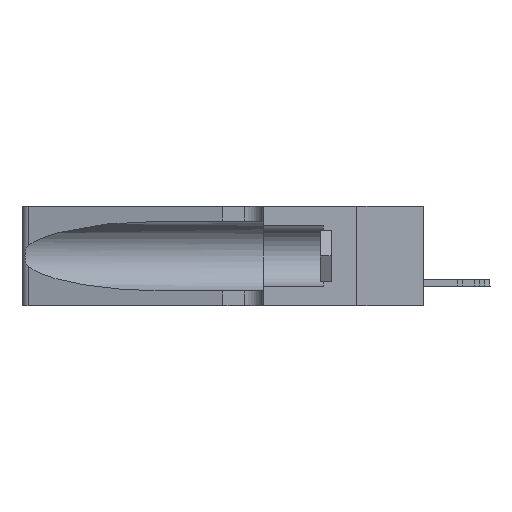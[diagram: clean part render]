
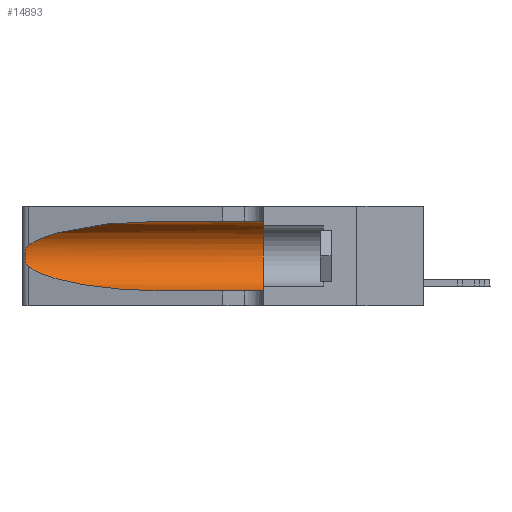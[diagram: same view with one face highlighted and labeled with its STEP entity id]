
A CAD part, left-side view. The second image highlights one B-rep face of the part: STEP entity #14893.
In plain terms, the highlighted cylindrical face has radius 3.308 mm (diameter 6.617 mm), a partial arc.
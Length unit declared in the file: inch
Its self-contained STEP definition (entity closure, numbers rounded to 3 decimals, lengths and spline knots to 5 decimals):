
#311 = ORIENTED_EDGE ( 'NONE', *, *, #1356, .T. ) ;
#380 = CARTESIAN_POINT ( 'NONE',  ( 0.1305, 1.61858, 0.185 ) ) ;
#923 = EDGE_CURVE ( 'NONE', #6857, #23272, #39423, .T. ) ;
#958 = VERTEX_POINT ( 'NONE', #23315 ) ;
#1293 = CARTESIAN_POINT ( 'NONE',  ( 0.25639, 1.23184, 0.21858 ) ) ;
#1356 = EDGE_CURVE ( 'NONE', #19249, #958, #8495, .T. ) ;
#1439 = CARTESIAN_POINT ( 'NONE',  ( 0.26018, 1.23835, 0.19895 ) ) ;
#3651 = CARTESIAN_POINT ( 'NONE',  ( 0.2373, 1.15595, 0.08982 ) ) ;
#4708 = CARTESIAN_POINT ( 'NONE',  ( 0.25787, 1.23484, 0.2124 ) ) ;
#4709 = ORIENTED_EDGE ( 'NONE', *, *, #27691, .F. ) ;
#4855 = CARTESIAN_POINT ( 'NONE',  ( 0.25856, 1.23593, 0.16098 ) ) ;
#5745 =( BOUNDED_CURVE ( )  B_SPLINE_CURVE ( 3, ( #30247, #43987, #16839, #43677 ),
 .UNSPECIFIED., .F., .F. ) 
 B_SPLINE_CURVE_WITH_KNOTS ( ( 4, 4 ),
 ( 1.5708, 2.84003 ),
 .UNSPECIFIED. ) 
 CURVE ( )  GEOMETRIC_REPRESENTATION_ITEM ( )  RATIONAL_B_SPLINE_CURVE ( ( 1., 0.87, 0.87, 1. ) ) 
 REPRESENTATION_ITEM ( '' )  );
#5772 = CYLINDRICAL_SURFACE ( 'NONE', #13787, 0.13025 ) ;
#6790 = CARTESIAN_POINT ( 'NONE',  ( 0.18966, 0.96281, 0.05475 ) ) ;
#6857 = VERTEX_POINT ( 'NONE', #15910 ) ;
#8495 =( BOUNDED_CURVE ( )  B_SPLINE_CURVE ( 3, ( #20632, #3651, #6790, #37813 ),
 .UNSPECIFIED., .F., .T. ) 
 B_SPLINE_CURVE_WITH_KNOTS ( ( 4, 4 ),
 ( 3.44316, 4.71239 ),
 .UNSPECIFIED. ) 
 CURVE ( )  GEOMETRIC_REPRESENTATION_ITEM ( )  RATIONAL_B_SPLINE_CURVE ( ( 1., 0.87, 0.87, 1. ) ) 
 REPRESENTATION_ITEM ( '' )  );
#10191 = CARTESIAN_POINT ( 'NONE',  ( 0.1305, 0.35, 0.05475 ) ) ;
#10659 = CARTESIAN_POINT ( 'NONE',  ( 0.25487, 1.22718, 0.22369 ) ) ;
#10666 = DIRECTION ( 'NONE',  ( 0., -1., 0. ) ) ;
#11580 = CARTESIAN_POINT ( 'NONE',  ( 0.26017, 1.23833, 0.17102 ) ) ;
#11704 = CARTESIAN_POINT ( 'NONE',  ( 0.25789, 1.23486, 0.15765 ) ) ;
#13498 = CARTESIAN_POINT ( 'NONE',  ( 0.1305, 1.61858, 0.05475 ) ) ;
#13705 = ORIENTED_EDGE ( 'NONE', *, *, #29795, .T. ) ;
#13787 = AXIS2_PLACEMENT_3D ( 'NONE', #380, #34554, #41704 ) ;
#13992 = CARTESIAN_POINT ( 'NONE',  ( 0.1305, 0.72297, 0.31525 ) ) ;
#14893 = ADVANCED_FACE ( 'NONE', ( #15908 ), #5772, .F. ) ;
#15137 = CARTESIAN_POINT ( 'NONE',  ( 0.25555, 1.22993, 0.14849 ) ) ;
#15287 = EDGE_LOOP ( 'NONE', ( #18714, #25810, #311, #13705, #36559, #4709 ) ) ;
#15363 = CARTESIAN_POINT ( 'NONE',  ( 0.1305, 1.61858, 0.31525 ) ) ;
#15885 = DIRECTION ( 'NONE',  ( 0., 1., 0. ) ) ;
#15908 = FACE_OUTER_BOUND ( 'NONE', #15287, .T. ) ;
#15910 = CARTESIAN_POINT ( 'NONE',  ( 0.1305, 0.35, 0.31525 ) ) ;
#15988 = EDGE_CURVE ( 'NONE', #28092, #32237, #5745, .T. ) ;
#16839 = CARTESIAN_POINT ( 'NONE',  ( 0.2373, 1.15595, 0.28018 ) ) ;
#18561 = CARTESIAN_POINT ( 'NONE',  ( 0.25487, 1.22718, 0.14631 ) ) ;
#18714 = ORIENTED_EDGE ( 'NONE', *, *, #15988, .T. ) ;
#19249 = VERTEX_POINT ( 'NONE', #23454 ) ;
#20632 = CARTESIAN_POINT ( 'NONE',  ( 0.25487, 1.22718, 0.14631 ) ) ;
#21546 = CARTESIAN_POINT ( 'NONE',  ( 0.26075, 1.23896, 0.19203 ) ) ;
#23272 = VERTEX_POINT ( 'NONE', #10191 ) ;
#23315 = CARTESIAN_POINT ( 'NONE',  ( 0.1305, 0.72297, 0.05475 ) ) ;
#23325 = VECTOR ( 'NONE', #39390, 39.37008 ) ;
#23454 = CARTESIAN_POINT ( 'NONE',  ( 0.25487, 1.22718, 0.14631 ) ) ;
#25810 = ORIENTED_EDGE ( 'NONE', *, *, #35422, .T. ) ;
#27691 = EDGE_CURVE ( 'NONE', #28092, #6857, #38302, .T. ) ;
#28092 = VERTEX_POINT ( 'NONE', #13992 ) ;
#29795 = EDGE_CURVE ( 'NONE', #958, #23272, #37540, .T. ) ;
#30247 = CARTESIAN_POINT ( 'NONE',  ( 0.1305, 0.72297, 0.31525 ) ) ;
#32150 = CARTESIAN_POINT ( 'NONE',  ( 0.26075, 1.23896, 0.178 ) ) ;
#32237 = VERTEX_POINT ( 'NONE', #10659 ) ;
#33364 = CARTESIAN_POINT ( 'NONE',  ( 0.1305, 0.35, 0.185 ) ) ;
#34554 = DIRECTION ( 'NONE',  ( 0., -1., 0. ) ) ;
#35422 = EDGE_CURVE ( 'NONE', #32237, #19249, #36121, .T. ) ;
#35585 = CARTESIAN_POINT ( 'NONE',  ( 0.25639, 1.23186, 0.15144 ) ) ;
#36121 = B_SPLINE_CURVE_WITH_KNOTS ( 'NONE', 3,
 ( #38412, #38571, #1293, #4708, #42003, #1439, #21546, #32150, #11580, #4855, #11704, #35585, #15137, #18561 ),
 .UNSPECIFIED., .F., .F.,
 ( 4, 2, 2, 2, 2, 2, 4 ),
 ( 0., 0.00027, 0.00053, 0.00107, 0.0016, 0.00187, 0.00214 ),
 .UNSPECIFIED. ) ;
#36559 = ORIENTED_EDGE ( 'NONE', *, *, #923, .F. ) ;
#37540 = LINE ( 'NONE', #13498, #43941 ) ;
#37813 = CARTESIAN_POINT ( 'NONE',  ( 0.1305, 0.72297, 0.05475 ) ) ;
#38302 = LINE ( 'NONE', #15363, #23325 ) ;
#38412 = CARTESIAN_POINT ( 'NONE',  ( 0.25487, 1.22718, 0.22369 ) ) ;
#38571 = CARTESIAN_POINT ( 'NONE',  ( 0.25555, 1.22994, 0.2215 ) ) ;
#39390 = DIRECTION ( 'NONE',  ( 0., -1., 0. ) ) ;
#39423 = CIRCLE ( 'NONE', #41727, 0.13025 ) ;
#39781 = DIRECTION ( 'NONE',  ( 0., 0., 1. ) ) ;
#41704 = DIRECTION ( 'NONE',  ( 0., 0., -1. ) ) ;
#41727 = AXIS2_PLACEMENT_3D ( 'NONE', #33364, #15885, #39781 ) ;
#42003 = CARTESIAN_POINT ( 'NONE',  ( 0.25854, 1.2359, 0.20912 ) ) ;
#43677 = CARTESIAN_POINT ( 'NONE',  ( 0.25487, 1.22718, 0.22369 ) ) ;
#43941 = VECTOR ( 'NONE', #10666, 39.37008 ) ;
#43987 = CARTESIAN_POINT ( 'NONE',  ( 0.18966, 0.96281, 0.31525 ) ) ;
